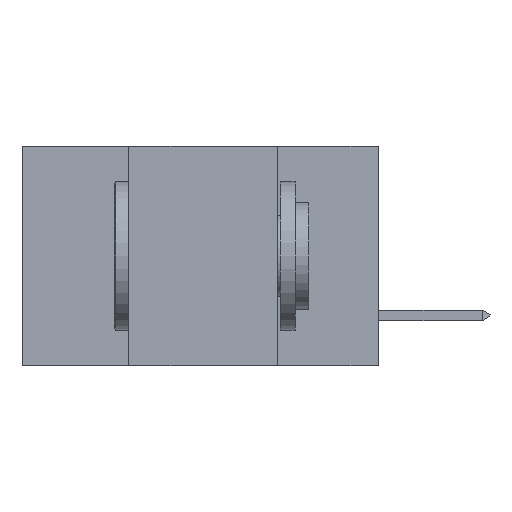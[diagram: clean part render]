
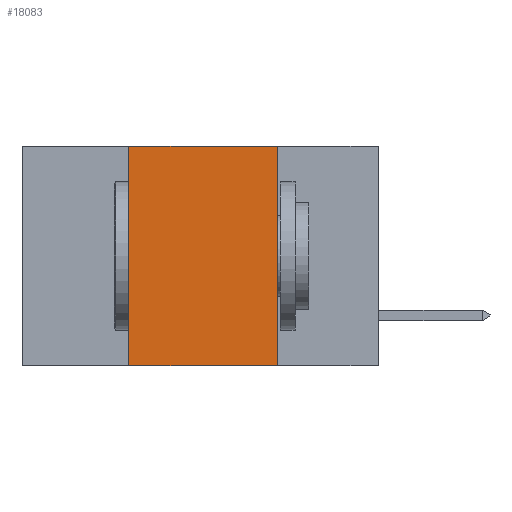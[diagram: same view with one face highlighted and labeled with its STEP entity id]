
A CAD part, left-side view. The second image highlights one B-rep face of the part: STEP entity #18083.
In plain terms, the highlighted planar face has unit normal (-1, 0, 0).
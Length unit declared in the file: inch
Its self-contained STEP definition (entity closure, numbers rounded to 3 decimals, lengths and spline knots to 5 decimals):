
#1531 = ORIENTED_EDGE ( 'NONE', *, *, #12555, .T. ) ;
#1892 = EDGE_CURVE ( 'NONE', #11714, #15621, #11348, .T. ) ;
#3239 = CARTESIAN_POINT ( 'NONE',  ( 0., 0.6, -0.37 ) ) ;
#4429 = ORIENTED_EDGE ( 'NONE', *, *, #11191, .F. ) ;
#6258 = VECTOR ( 'NONE', #21358, 39.37008 ) ;
#6990 = VERTEX_POINT ( 'NONE', #11726 ) ;
#7405 = AXIS2_PLACEMENT_3D ( 'NONE', #16850, #21798, #18472 ) ;
#7784 = EDGE_CURVE ( 'NONE', #19114, #6990, #15011, .T. ) ;
#9732 = PLANE ( 'NONE',  #7405 ) ;
#10252 = DIRECTION ( 'NONE',  ( 0., -1., 0. ) ) ;
#10579 = ORIENTED_EDGE ( 'NONE', *, *, #7784, .F. ) ;
#11191 = EDGE_CURVE ( 'NONE', #6990, #11714, #18658, .T. ) ;
#11348 = LINE ( 'NONE', #14337, #6258 ) ;
#11525 = DIRECTION ( 'NONE',  ( 0., -1., 0. ) ) ;
#11714 = VERTEX_POINT ( 'NONE', #12065 ) ;
#11726 = CARTESIAN_POINT ( 'NONE',  ( 0., 0.42, 0. ) ) ;
#12065 = CARTESIAN_POINT ( 'NONE',  ( 0., 0.17, 0. ) ) ;
#12555 = EDGE_CURVE ( 'NONE', #19114, #15621, #19009, .T. ) ;
#13831 = VECTOR ( 'NONE', #10252, 39.37008 ) ;
#14337 = CARTESIAN_POINT ( 'NONE',  ( 0., 0.17, -0.37 ) ) ;
#15011 = LINE ( 'NONE', #15124, #15204 ) ;
#15124 = CARTESIAN_POINT ( 'NONE',  ( 0., 0.42, -0.37 ) ) ;
#15204 = VECTOR ( 'NONE', #22255, 39.37008 ) ;
#15515 = ORIENTED_EDGE ( 'NONE', *, *, #1892, .F. ) ;
#15621 = VERTEX_POINT ( 'NONE', #22671 ) ;
#16164 = CARTESIAN_POINT ( 'NONE',  ( 0., 0.42, -0.37 ) ) ;
#16738 = VECTOR ( 'NONE', #11525, 39.37008 ) ;
#16850 = CARTESIAN_POINT ( 'NONE',  ( 0., 0.6, 0. ) ) ;
#16967 = FACE_OUTER_BOUND ( 'NONE', #21714, .T. ) ;
#18083 = ADVANCED_FACE ( 'NONE', ( #16967 ), #9732, .F. ) ;
#18472 = DIRECTION ( 'NONE',  ( 0., 0., -1. ) ) ;
#18658 = LINE ( 'NONE', #21883, #16738 ) ;
#19009 = LINE ( 'NONE', #3239, #13831 ) ;
#19114 = VERTEX_POINT ( 'NONE', #16164 ) ;
#21358 = DIRECTION ( 'NONE',  ( 0., 0., -1. ) ) ;
#21714 = EDGE_LOOP ( 'NONE', ( #15515, #4429, #10579, #1531 ) ) ;
#21798 = DIRECTION ( 'NONE',  ( 1., 0., 0. ) ) ;
#21883 = CARTESIAN_POINT ( 'NONE',  ( 0., 0.6, 0. ) ) ;
#22255 = DIRECTION ( 'NONE',  ( 0., 0., 1. ) ) ;
#22671 = CARTESIAN_POINT ( 'NONE',  ( 0., 0.17, -0.37 ) ) ;
